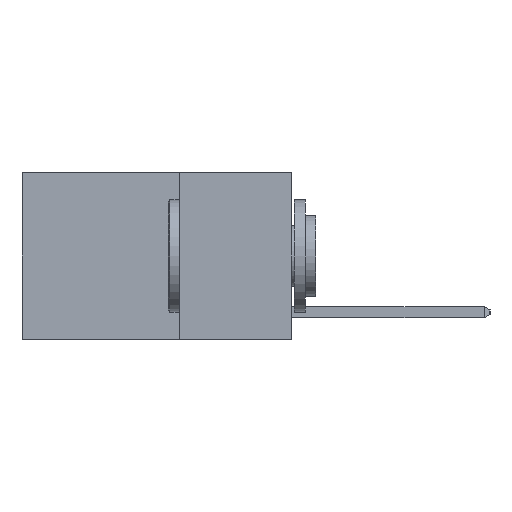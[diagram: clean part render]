
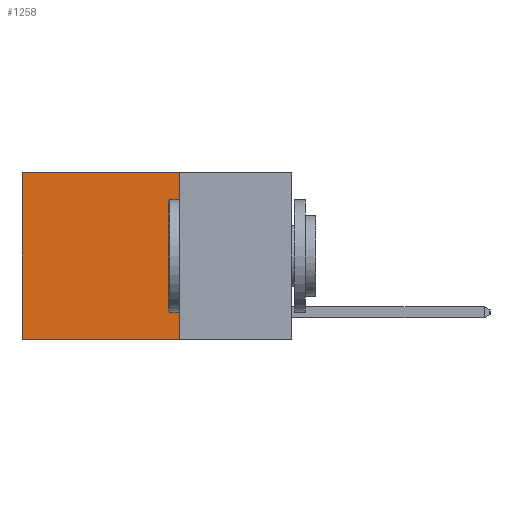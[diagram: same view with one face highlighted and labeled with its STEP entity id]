
A CAD part, left-side view. The second image highlights one B-rep face of the part: STEP entity #1258.
In plain terms, the highlighted planar face has unit normal (-1, 0, 0).
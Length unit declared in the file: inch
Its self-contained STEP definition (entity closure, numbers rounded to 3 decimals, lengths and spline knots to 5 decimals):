
#417 = DIRECTION ( 'NONE',  ( 0., 1., 0. ) ) ;
#851 = VECTOR ( 'NONE', #9263, 39.37008 ) ;
#1148 = LINE ( 'NONE', #8349, #851 ) ;
#1258 = ADVANCED_FACE ( 'NONE', ( #7697 ), #2600, .F. ) ;
#1516 = VECTOR ( 'NONE', #417, 39.37008 ) ;
#1660 = VERTEX_POINT ( 'NONE', #10116 ) ;
#2116 = EDGE_LOOP ( 'NONE', ( #5476, #9627, #7108, #7671 ) ) ;
#2584 = DIRECTION ( 'NONE',  ( 0., 0., -1. ) ) ;
#2589 = DIRECTION ( 'NONE',  ( 1., 0., 0. ) ) ;
#2600 = PLANE ( 'NONE',  #2808 ) ;
#2781 = CARTESIAN_POINT ( 'NONE',  ( 0.2625, 0.25, 0. ) ) ;
#2808 = AXIS2_PLACEMENT_3D ( 'NONE', #2781, #2589, #2584 ) ;
#3571 = EDGE_CURVE ( 'NONE', #8205, #4406, #9055, .T. ) ;
#4159 = CARTESIAN_POINT ( 'NONE',  ( 0.2625, 0.25, 0. ) ) ;
#4231 = VECTOR ( 'NONE', #9616, 39.37008 ) ;
#4293 = CARTESIAN_POINT ( 'NONE',  ( 0.2625, 0.6, -0.37 ) ) ;
#4406 = VERTEX_POINT ( 'NONE', #4293 ) ;
#4857 = VERTEX_POINT ( 'NONE', #4159 ) ;
#5476 = ORIENTED_EDGE ( 'NONE', *, *, #8966, .T. ) ;
#7108 = ORIENTED_EDGE ( 'NONE', *, *, #9118, .F. ) ;
#7671 = ORIENTED_EDGE ( 'NONE', *, *, #11367, .T. ) ;
#7697 = FACE_OUTER_BOUND ( 'NONE', #2116, .T. ) ;
#7829 = CARTESIAN_POINT ( 'NONE',  ( 0.2625, 0.25, 0. ) ) ;
#8205 = VERTEX_POINT ( 'NONE', #11450 ) ;
#8349 = CARTESIAN_POINT ( 'NONE',  ( 0.2625, 0.25, 0. ) ) ;
#8966 = EDGE_CURVE ( 'NONE', #1660, #4406, #9539, .T. ) ;
#9055 = LINE ( 'NONE', #9502, #1516 ) ;
#9101 = CARTESIAN_POINT ( 'NONE',  ( 0.2625, 0.6, 0. ) ) ;
#9118 = EDGE_CURVE ( 'NONE', #4857, #8205, #1148, .T. ) ;
#9263 = DIRECTION ( 'NONE',  ( 0., 0., -1. ) ) ;
#9265 = VECTOR ( 'NONE', #10887, 39.37008 ) ;
#9502 = CARTESIAN_POINT ( 'NONE',  ( 0.2625, 0.25, -0.37 ) ) ;
#9539 = LINE ( 'NONE', #9101, #9265 ) ;
#9616 = DIRECTION ( 'NONE',  ( 0., 1., 0. ) ) ;
#9627 = ORIENTED_EDGE ( 'NONE', *, *, #3571, .F. ) ;
#10116 = CARTESIAN_POINT ( 'NONE',  ( 0.2625, 0.6, 0. ) ) ;
#10887 = DIRECTION ( 'NONE',  ( 0., 0., -1. ) ) ;
#11367 = EDGE_CURVE ( 'NONE', #4857, #1660, #11390, .T. ) ;
#11390 = LINE ( 'NONE', #7829, #4231 ) ;
#11450 = CARTESIAN_POINT ( 'NONE',  ( 0.2625, 0.25, -0.37 ) ) ;
